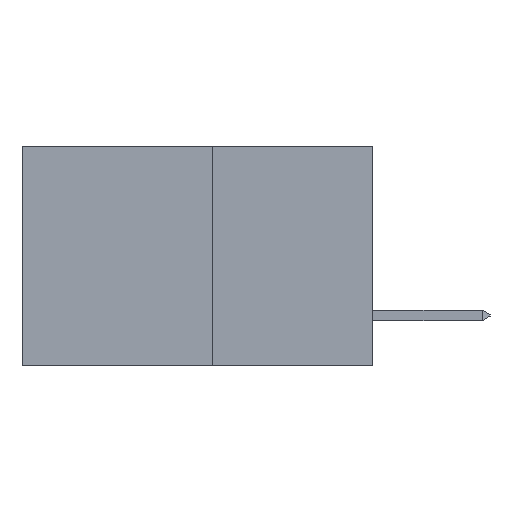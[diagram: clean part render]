
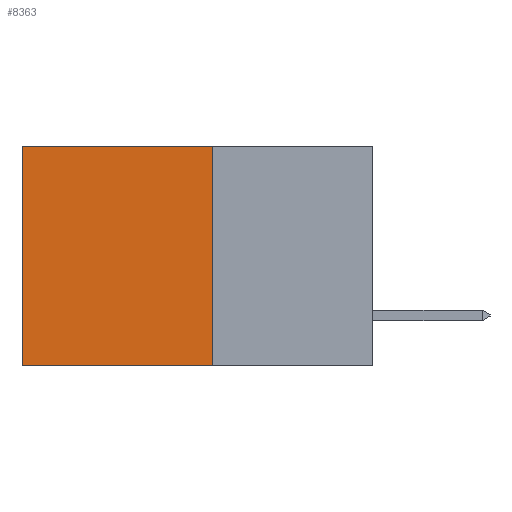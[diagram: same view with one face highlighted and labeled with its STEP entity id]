
A CAD part, left-side view. The second image highlights one B-rep face of the part: STEP entity #8363.
In plain terms, the highlighted planar face has unit normal (-1, 0, 0).
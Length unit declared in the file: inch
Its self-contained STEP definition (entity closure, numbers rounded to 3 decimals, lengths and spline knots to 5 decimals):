
#348 = VERTEX_POINT ( 'NONE', #9914 ) ;
#644 = EDGE_CURVE ( 'NONE', #348, #8878, #9115, .T. ) ;
#1225 = VECTOR ( 'NONE', #3892, 39.37008 ) ;
#1925 = VERTEX_POINT ( 'NONE', #13484 ) ;
#2358 = CARTESIAN_POINT ( 'NONE',  ( 0.277, 0.27, -0.37 ) ) ;
#2545 = VECTOR ( 'NONE', #7735, 39.37008 ) ;
#3837 = ORIENTED_EDGE ( 'NONE', *, *, #12829, .T. ) ;
#3892 = DIRECTION ( 'NONE',  ( 0., 0., -1. ) ) ;
#4532 = DIRECTION ( 'NONE',  ( 0., 1., 0. ) ) ;
#4588 = CARTESIAN_POINT ( 'NONE',  ( 0.277, 0.27, 0. ) ) ;
#4806 = EDGE_CURVE ( 'NONE', #348, #17405, #15778, .T. ) ;
#4996 = VECTOR ( 'NONE', #4532, 39.37008 ) ;
#5490 = CARTESIAN_POINT ( 'NONE',  ( 0.277, 0.59, -0.37 ) ) ;
#5860 = ORIENTED_EDGE ( 'NONE', *, *, #4806, .T. ) ;
#7387 = DIRECTION ( 'NONE',  ( 0., 0., -1. ) ) ;
#7397 = AXIS2_PLACEMENT_3D ( 'NONE', #7413, #7408, #7387 ) ;
#7408 = DIRECTION ( 'NONE',  ( 1., 0., 0. ) ) ;
#7413 = CARTESIAN_POINT ( 'NONE',  ( 0.277, 0.27, -0.37 ) ) ;
#7458 = ORIENTED_EDGE ( 'NONE', *, *, #644, .F. ) ;
#7539 = EDGE_CURVE ( 'NONE', #8878, #1925, #10314, .T. ) ;
#7735 = DIRECTION ( 'NONE',  ( 0., 1., 0. ) ) ;
#7864 = PLANE ( 'NONE',  #7397 ) ;
#8363 = ADVANCED_FACE ( 'NONE', ( #17435 ), #7864, .F. ) ;
#8878 = VERTEX_POINT ( 'NONE', #2358 ) ;
#8897 = CARTESIAN_POINT ( 'NONE',  ( 0.277, 0.27, -0.37 ) ) ;
#9115 = LINE ( 'NONE', #9743, #1225 ) ;
#9743 = CARTESIAN_POINT ( 'NONE',  ( 0.277, 0.27, -0.37 ) ) ;
#9914 = CARTESIAN_POINT ( 'NONE',  ( 0.277, 0.27, 0. ) ) ;
#10314 = LINE ( 'NONE', #8897, #2545 ) ;
#10794 = ORIENTED_EDGE ( 'NONE', *, *, #7539, .F. ) ;
#12829 = EDGE_CURVE ( 'NONE', #17405, #1925, #14665, .T. ) ;
#13484 = CARTESIAN_POINT ( 'NONE',  ( 0.277, 0.59, -0.37 ) ) ;
#13857 = EDGE_LOOP ( 'NONE', ( #3837, #10794, #7458, #5860 ) ) ;
#14665 = LINE ( 'NONE', #5490, #15076 ) ;
#14936 = DIRECTION ( 'NONE',  ( 0., 0., -1. ) ) ;
#15076 = VECTOR ( 'NONE', #14936, 39.37008 ) ;
#15778 = LINE ( 'NONE', #4588, #4996 ) ;
#17063 = CARTESIAN_POINT ( 'NONE',  ( 0.277, 0.59, 0. ) ) ;
#17405 = VERTEX_POINT ( 'NONE', #17063 ) ;
#17435 = FACE_OUTER_BOUND ( 'NONE', #13857, .T. ) ;
